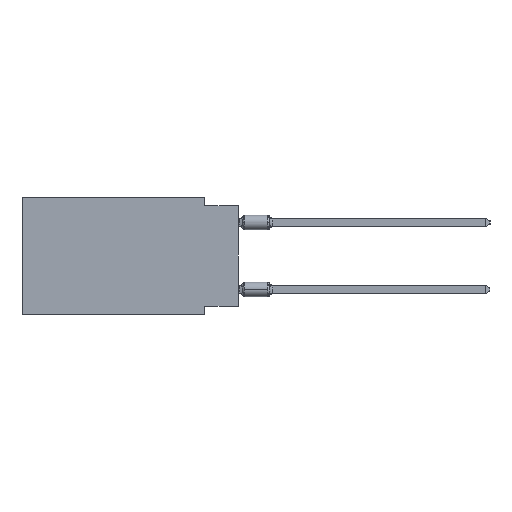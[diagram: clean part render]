
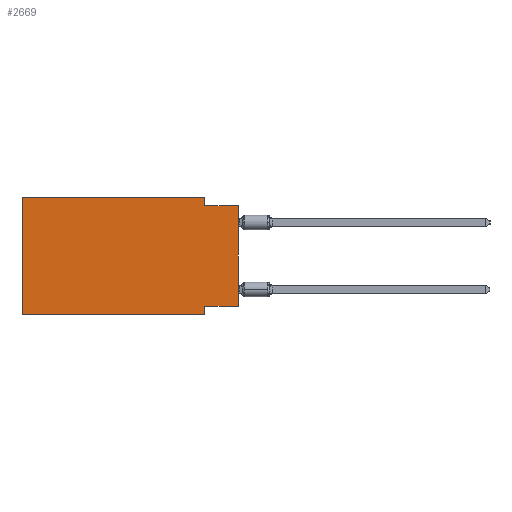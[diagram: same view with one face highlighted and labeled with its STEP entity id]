
A CAD part, left-side view. The second image highlights one B-rep face of the part: STEP entity #2669.
In plain terms, the highlighted planar face has unit normal (-1, 0, 0).
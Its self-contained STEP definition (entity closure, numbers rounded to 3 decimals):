
#225 = EDGE_CURVE ( 'NONE', #863, #11614, #11083, .T. ) ;
#267 = DIRECTION ( 'NONE',  ( 0., 1., 0. ) ) ;
#863 = VERTEX_POINT ( 'NONE', #9553 ) ;
#887 = DIRECTION ( 'NONE',  ( 0., 0., 1. ) ) ;
#1078 = VECTOR ( 'NONE', #8200, 1000. ) ;
#1100 = CARTESIAN_POINT ( 'NONE',  ( 0., 16.383, 0. ) ) ;
#1167 = CARTESIAN_POINT ( 'NONE',  ( 0., 2.54, -8.89 ) ) ;
#1526 = EDGE_CURVE ( 'NONE', #6518, #11614, #5204, .T. ) ;
#1773 = CARTESIAN_POINT ( 'NONE',  ( 0., 2.54, -8.255 ) ) ;
#1777 = ORIENTED_EDGE ( 'NONE', *, *, #10271, .F. ) ;
#2176 = CARTESIAN_POINT ( 'NONE',  ( 0., 16.383, 0. ) ) ;
#2320 = CARTESIAN_POINT ( 'NONE',  ( 0., 2.54, 0. ) ) ;
#2669 = ADVANCED_FACE ( 'NONE', ( #6305 ), #17584, .F. ) ;
#3489 = DIRECTION ( 'NONE',  ( 1., 0., 0. ) ) ;
#3716 = CARTESIAN_POINT ( 'NONE',  ( 0., 2.54, -0.635 ) ) ;
#3818 = VERTEX_POINT ( 'NONE', #13453 ) ;
#3927 = CARTESIAN_POINT ( 'NONE',  ( 0., 2.54, -8.89 ) ) ;
#4739 = ORIENTED_EDGE ( 'NONE', *, *, #11609, .F. ) ;
#5204 = LINE ( 'NONE', #1167, #9157 ) ;
#5393 = VERTEX_POINT ( 'NONE', #2320 ) ;
#5471 = ORIENTED_EDGE ( 'NONE', *, *, #11359, .T. ) ;
#6271 = EDGE_CURVE ( 'NONE', #863, #9949, #13335, .T. ) ;
#6305 = FACE_OUTER_BOUND ( 'NONE', #11420, .T. ) ;
#6518 = VERTEX_POINT ( 'NONE', #1773 ) ;
#6754 = DIRECTION ( 'NONE',  ( 0., 0., -1. ) ) ;
#6756 = EDGE_CURVE ( 'NONE', #9949, #5393, #16866, .T. ) ;
#6853 = CARTESIAN_POINT ( 'NONE',  ( 0., 16.383, -8.89 ) ) ;
#7113 = DIRECTION ( 'NONE',  ( 0., -1., 0. ) ) ;
#7330 = VECTOR ( 'NONE', #267, 1000. ) ;
#7487 = VECTOR ( 'NONE', #11994, 1000. ) ;
#8200 = DIRECTION ( 'NONE',  ( 0., 0., 1. ) ) ;
#8241 = LINE ( 'NONE', #8424, #15676 ) ;
#8371 = LINE ( 'NONE', #10923, #1078 ) ;
#8424 = CARTESIAN_POINT ( 'NONE',  ( 0., 0., -0.635 ) ) ;
#9157 = VECTOR ( 'NONE', #6754, 1000. ) ;
#9211 = ORIENTED_EDGE ( 'NONE', *, *, #6271, .F. ) ;
#9553 = CARTESIAN_POINT ( 'NONE',  ( 0., 16.383, -8.89 ) ) ;
#9855 = ORIENTED_EDGE ( 'NONE', *, *, #6756, .F. ) ;
#9949 = VERTEX_POINT ( 'NONE', #1100 ) ;
#9957 = VERTEX_POINT ( 'NONE', #17603 ) ;
#10271 = EDGE_CURVE ( 'NONE', #9957, #6518, #13089, .T. ) ;
#10885 = CARTESIAN_POINT ( 'NONE',  ( 0., 2.54, 0. ) ) ;
#10923 = CARTESIAN_POINT ( 'NONE',  ( 0., 0., 0. ) ) ;
#11083 = LINE ( 'NONE', #6853, #15398 ) ;
#11359 = EDGE_CURVE ( 'NONE', #9957, #3818, #8371, .T. ) ;
#11420 = EDGE_LOOP ( 'NONE', ( #5471, #14661, #4739, #9855, #9211, #16518, #16914, #1777 ) ) ;
#11609 = EDGE_CURVE ( 'NONE', #5393, #17815, #13624, .T. ) ;
#11614 = VERTEX_POINT ( 'NONE', #3927 ) ;
#11699 = EDGE_CURVE ( 'NONE', #17815, #3818, #8241, .T. ) ;
#11994 = DIRECTION ( 'NONE',  ( 0., 0., -1. ) ) ;
#12156 = DIRECTION ( 'NONE',  ( 0., 0., -1. ) ) ;
#12777 = VECTOR ( 'NONE', #14098, 1000. ) ;
#13089 = LINE ( 'NONE', #14286, #7330 ) ;
#13335 = LINE ( 'NONE', #2176, #16312 ) ;
#13453 = CARTESIAN_POINT ( 'NONE',  ( 0., 0., -0.635 ) ) ;
#13529 = CARTESIAN_POINT ( 'NONE',  ( 0., 16.383, 0. ) ) ;
#13624 = LINE ( 'NONE', #10885, #7487 ) ;
#14098 = DIRECTION ( 'NONE',  ( 0., -1., 0. ) ) ;
#14286 = CARTESIAN_POINT ( 'NONE',  ( 0., 0., -8.255 ) ) ;
#14661 = ORIENTED_EDGE ( 'NONE', *, *, #11699, .F. ) ;
#14954 = DIRECTION ( 'NONE',  ( 0., -1., 0. ) ) ;
#15385 = CARTESIAN_POINT ( 'NONE',  ( 0., 16.383, 0. ) ) ;
#15398 = VECTOR ( 'NONE', #14954, 1000. ) ;
#15676 = VECTOR ( 'NONE', #7113, 1000. ) ;
#16194 = AXIS2_PLACEMENT_3D ( 'NONE', #13529, #3489, #12156 ) ;
#16312 = VECTOR ( 'NONE', #887, 1000. ) ;
#16518 = ORIENTED_EDGE ( 'NONE', *, *, #225, .T. ) ;
#16866 = LINE ( 'NONE', #15385, #12777 ) ;
#16914 = ORIENTED_EDGE ( 'NONE', *, *, #1526, .F. ) ;
#17584 = PLANE ( 'NONE',  #16194 ) ;
#17603 = CARTESIAN_POINT ( 'NONE',  ( 0., 0., -8.255 ) ) ;
#17815 = VERTEX_POINT ( 'NONE', #3716 ) ;
